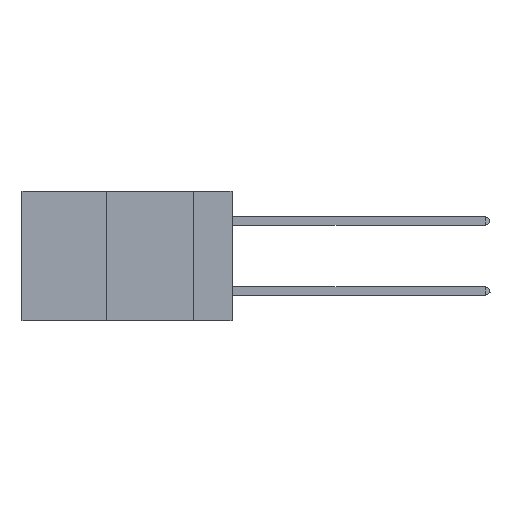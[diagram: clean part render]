
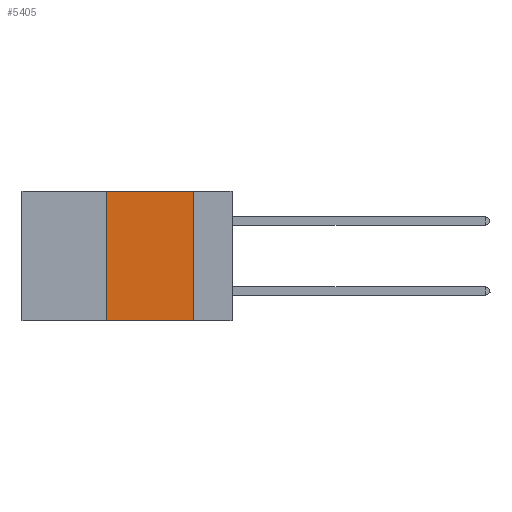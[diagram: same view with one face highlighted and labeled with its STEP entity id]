
A CAD part, left-side view. The second image highlights one B-rep face of the part: STEP entity #5405.
In plain terms, the highlighted planar face has unit normal (-1, 0, 0).
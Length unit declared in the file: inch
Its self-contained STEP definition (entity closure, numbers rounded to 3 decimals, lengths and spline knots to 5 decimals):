
#65 = VECTOR ( 'NONE', #16832, 39.37008 ) ;
#207 = CARTESIAN_POINT ( 'NONE',  ( 0., 0.11, 0. ) ) ;
#303 = ORIENTED_EDGE ( 'NONE', *, *, #14023, .F. ) ;
#393 = ORIENTED_EDGE ( 'NONE', *, *, #18259, .T. ) ;
#608 = CARTESIAN_POINT ( 'NONE',  ( 0., 0.36, 0. ) ) ;
#2546 = EDGE_CURVE ( 'NONE', #19340, #5177, #3881, .T. ) ;
#3265 = DIRECTION ( 'NONE',  ( 1., 0., 0. ) ) ;
#3390 = CARTESIAN_POINT ( 'NONE',  ( 0., 0.36, -0.37 ) ) ;
#3881 = LINE ( 'NONE', #10817, #5377 ) ;
#5177 = VERTEX_POINT ( 'NONE', #5921 ) ;
#5377 = VECTOR ( 'NONE', #16979, 39.37008 ) ;
#5405 = ADVANCED_FACE ( 'NONE', ( #20470 ), #12805, .F. ) ;
#5921 = CARTESIAN_POINT ( 'NONE',  ( 0., 0.11, 0. ) ) ;
#6373 = CARTESIAN_POINT ( 'NONE',  ( 0., 0.36, 0. ) ) ;
#7822 = LINE ( 'NONE', #207, #14071 ) ;
#7952 = DIRECTION ( 'NONE',  ( 0., 0., -1. ) ) ;
#9182 = DIRECTION ( 'NONE',  ( 0., -1., 0. ) ) ;
#10484 = VERTEX_POINT ( 'NONE', #19538 ) ;
#10817 = CARTESIAN_POINT ( 'NONE',  ( 0., 0.6, 0. ) ) ;
#11181 = ORIENTED_EDGE ( 'NONE', *, *, #2546, .F. ) ;
#11685 = DIRECTION ( 'NONE',  ( 0., 0., -1. ) ) ;
#12134 = CARTESIAN_POINT ( 'NONE',  ( 0., 0.6, -0.37 ) ) ;
#12805 = PLANE ( 'NONE',  #12811 ) ;
#12811 = AXIS2_PLACEMENT_3D ( 'NONE', #12877, #3265, #11685 ) ;
#12877 = CARTESIAN_POINT ( 'NONE',  ( 0., 0.6, 0. ) ) ;
#13984 = LINE ( 'NONE', #608, #65 ) ;
#14023 = EDGE_CURVE ( 'NONE', #18567, #19340, #13984, .T. ) ;
#14071 = VECTOR ( 'NONE', #7952, 39.37008 ) ;
#15300 = LINE ( 'NONE', #12134, #17544 ) ;
#16832 = DIRECTION ( 'NONE',  ( 0., 0., 1. ) ) ;
#16979 = DIRECTION ( 'NONE',  ( 0., -1., 0. ) ) ;
#17544 = VECTOR ( 'NONE', #9182, 39.37008 ) ;
#17707 = EDGE_CURVE ( 'NONE', #5177, #10484, #7822, .T. ) ;
#18259 = EDGE_CURVE ( 'NONE', #18567, #10484, #15300, .T. ) ;
#18567 = VERTEX_POINT ( 'NONE', #3390 ) ;
#18627 = ORIENTED_EDGE ( 'NONE', *, *, #17707, .F. ) ;
#19340 = VERTEX_POINT ( 'NONE', #6373 ) ;
#19538 = CARTESIAN_POINT ( 'NONE',  ( 0., 0.11, -0.37 ) ) ;
#19564 = EDGE_LOOP ( 'NONE', ( #18627, #11181, #303, #393 ) ) ;
#20470 = FACE_OUTER_BOUND ( 'NONE', #19564, .T. ) ;
